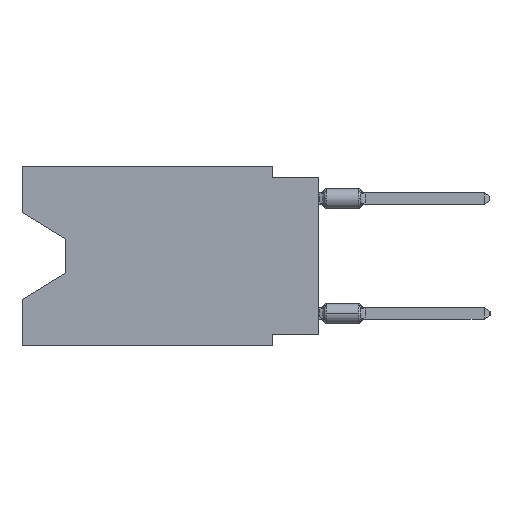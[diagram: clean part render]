
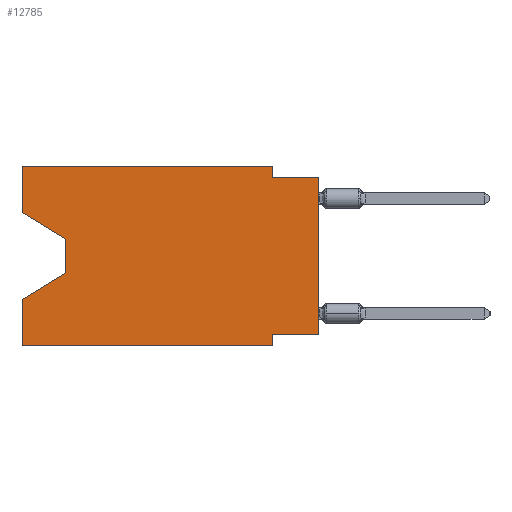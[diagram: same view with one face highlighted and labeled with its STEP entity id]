
A CAD part, left-side view. The second image highlights one B-rep face of the part: STEP entity #12785.
In plain terms, the highlighted planar face has unit normal (-1, 0, 0).
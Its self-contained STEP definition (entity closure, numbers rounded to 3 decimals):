
#31 = LINE ( 'NONE', #40084, #26179 ) ;
#1587 = VECTOR ( 'NONE', #42313, 1000. ) ;
#1826 = ORIENTED_EDGE ( 'NONE', *, *, #6703, .F. ) ;
#2196 = VERTEX_POINT ( 'NONE', #48618 ) ;
#2496 = VERTEX_POINT ( 'NONE', #7044 ) ;
#2549 = VERTEX_POINT ( 'NONE', #28681 ) ;
#4661 = DIRECTION ( 'NONE',  ( 0., -1., 0. ) ) ;
#5457 = ORIENTED_EDGE ( 'NONE', *, *, #55264, .T. ) ;
#5834 = DIRECTION ( 'NONE',  ( 0., 0., 1. ) ) ;
#6442 = VECTOR ( 'NONE', #52381, 1000. ) ;
#6459 = LINE ( 'NONE', #33902, #17753 ) ;
#6703 = EDGE_CURVE ( 'NONE', #23717, #7166, #6459, .T. ) ;
#6745 = DIRECTION ( 'NONE',  ( 0., -1., 0. ) ) ;
#7044 = CARTESIAN_POINT ( 'NONE',  ( 0., 0., -9.271 ) ) ;
#7166 = VERTEX_POINT ( 'NONE', #23918 ) ;
#8483 = LINE ( 'NONE', #8770, #37005 ) ;
#8770 = CARTESIAN_POINT ( 'NONE',  ( 0., 16.383, -9.906 ) ) ;
#9251 = DIRECTION ( 'NONE',  ( 0., -1., 0. ) ) ;
#9949 = VECTOR ( 'NONE', #29455, 1000. ) ;
#10084 = CARTESIAN_POINT ( 'NONE',  ( 0., 2.54, -9.271 ) ) ;
#10086 = ORIENTED_EDGE ( 'NONE', *, *, #16750, .F. ) ;
#10589 = ORIENTED_EDGE ( 'NONE', *, *, #33788, .F. ) ;
#11065 = ORIENTED_EDGE ( 'NONE', *, *, #12169, .T. ) ;
#11850 = VERTEX_POINT ( 'NONE', #42985 ) ;
#12040 = EDGE_CURVE ( 'NONE', #2496, #49996, #18697, .T. ) ;
#12117 = EDGE_CURVE ( 'NONE', #20123, #30701, #14608, .T. ) ;
#12169 = EDGE_CURVE ( 'NONE', #35617, #2549, #37944, .T. ) ;
#12319 = DIRECTION ( 'NONE',  ( 0., -0.855, -0.519 ) ) ;
#12782 = EDGE_CURVE ( 'NONE', #2496, #46927, #25050, .T. ) ;
#12785 = ADVANCED_FACE ( 'NONE', ( #55509 ), #16296, .F. ) ;
#14608 = LINE ( 'NONE', #41763, #45422 ) ;
#15513 = CARTESIAN_POINT ( 'NONE',  ( 0., 16.383, 0. ) ) ;
#16296 = PLANE ( 'NONE',  #34241 ) ;
#16750 = EDGE_CURVE ( 'NONE', #46927, #11850, #44417, .T. ) ;
#17237 = CARTESIAN_POINT ( 'NONE',  ( 0., 2.54, -0.635 ) ) ;
#17753 = VECTOR ( 'NONE', #6745, 1000. ) ;
#18697 = LINE ( 'NONE', #54401, #20220 ) ;
#19519 = DIRECTION ( 'NONE',  ( 1., 0., 0. ) ) ;
#20123 = VERTEX_POINT ( 'NONE', #31411 ) ;
#20220 = VECTOR ( 'NONE', #5834, 1000. ) ;
#20280 = EDGE_CURVE ( 'NONE', #7166, #43004, #31, .T. ) ;
#20502 = LINE ( 'NONE', #48001, #32930 ) ;
#22540 = EDGE_CURVE ( 'NONE', #2196, #23717, #42379, .T. ) ;
#23717 = VERTEX_POINT ( 'NONE', #15513 ) ;
#23875 = ORIENTED_EDGE ( 'NONE', *, *, #20280, .F. ) ;
#23899 = CARTESIAN_POINT ( 'NONE',  ( 0., 16.383, 0. ) ) ;
#23918 = CARTESIAN_POINT ( 'NONE',  ( 0., 2.54, 0. ) ) ;
#24478 = DIRECTION ( 'NONE',  ( 0., 0., -1. ) ) ;
#24579 = EDGE_CURVE ( 'NONE', #2196, #35617, #20502, .T. ) ;
#25050 = LINE ( 'NONE', #42595, #1587 ) ;
#25180 = CARTESIAN_POINT ( 'NONE',  ( 0., 16.383, -7.36 ) ) ;
#26179 = VECTOR ( 'NONE', #44776, 1000. ) ;
#28681 = CARTESIAN_POINT ( 'NONE',  ( 0., 13.97, -5.893 ) ) ;
#29258 = VECTOR ( 'NONE', #9251, 1000. ) ;
#29455 = DIRECTION ( 'NONE',  ( 0., 0., -1. ) ) ;
#30701 = VERTEX_POINT ( 'NONE', #25180 ) ;
#30786 = ORIENTED_EDGE ( 'NONE', *, *, #12117, .F. ) ;
#31411 = CARTESIAN_POINT ( 'NONE',  ( 0., 16.383, -9.906 ) ) ;
#32930 = VECTOR ( 'NONE', #12319, 1000. ) ;
#33788 = EDGE_CURVE ( 'NONE', #43004, #49996, #49308, .T. ) ;
#33902 = CARTESIAN_POINT ( 'NONE',  ( 0., 16.383, 0. ) ) ;
#34241 = AXIS2_PLACEMENT_3D ( 'NONE', #23899, #19519, #24478 ) ;
#34462 = DIRECTION ( 'NONE',  ( 0., 0., 1. ) ) ;
#35617 = VERTEX_POINT ( 'NONE', #55090 ) ;
#37005 = VECTOR ( 'NONE', #4661, 1000. ) ;
#37944 = LINE ( 'NONE', #43214, #9949 ) ;
#38611 = LINE ( 'NONE', #38900, #6442 ) ;
#38900 = CARTESIAN_POINT ( 'NONE',  ( 0., 13.97, -5.893 ) ) ;
#39990 = ORIENTED_EDGE ( 'NONE', *, *, #12782, .F. ) ;
#40084 = CARTESIAN_POINT ( 'NONE',  ( 0., 2.54, 0. ) ) ;
#40630 = DIRECTION ( 'NONE',  ( 0., 0., 1. ) ) ;
#41763 = CARTESIAN_POINT ( 'NONE',  ( 0., 16.383, 0. ) ) ;
#42313 = DIRECTION ( 'NONE',  ( 0., 1., 0. ) ) ;
#42379 = LINE ( 'NONE', #43250, #44149 ) ;
#42595 = CARTESIAN_POINT ( 'NONE',  ( 0., 0., -9.271 ) ) ;
#42985 = CARTESIAN_POINT ( 'NONE',  ( 0., 2.54, -9.906 ) ) ;
#43004 = VERTEX_POINT ( 'NONE', #17237 ) ;
#43214 = CARTESIAN_POINT ( 'NONE',  ( 0., 13.97, -4.013 ) ) ;
#43250 = CARTESIAN_POINT ( 'NONE',  ( 0., 16.383, 0. ) ) ;
#44149 = VECTOR ( 'NONE', #34462, 1000. ) ;
#44417 = LINE ( 'NONE', #48528, #51289 ) ;
#44776 = DIRECTION ( 'NONE',  ( 0., 0., -1. ) ) ;
#45422 = VECTOR ( 'NONE', #40630, 1000. ) ;
#46927 = VERTEX_POINT ( 'NONE', #10084 ) ;
#47626 = EDGE_CURVE ( 'NONE', #2549, #30701, #38611, .T. ) ;
#48001 = CARTESIAN_POINT ( 'NONE',  ( 0., 16.383, -2.546 ) ) ;
#48528 = CARTESIAN_POINT ( 'NONE',  ( 0., 2.54, -9.906 ) ) ;
#48618 = CARTESIAN_POINT ( 'NONE',  ( 0., 16.383, -2.546 ) ) ;
#49308 = LINE ( 'NONE', #57515, #29258 ) ;
#49441 = ORIENTED_EDGE ( 'NONE', *, *, #24579, .T. ) ;
#49641 = ORIENTED_EDGE ( 'NONE', *, *, #12040, .T. ) ;
#49996 = VERTEX_POINT ( 'NONE', #51877 ) ;
#51289 = VECTOR ( 'NONE', #53798, 1000. ) ;
#51636 = ORIENTED_EDGE ( 'NONE', *, *, #47626, .T. ) ;
#51877 = CARTESIAN_POINT ( 'NONE',  ( 0., 0., -0.635 ) ) ;
#52381 = DIRECTION ( 'NONE',  ( 0., 0.855, -0.519 ) ) ;
#53798 = DIRECTION ( 'NONE',  ( 0., 0., -1. ) ) ;
#54401 = CARTESIAN_POINT ( 'NONE',  ( 0., 0., 0. ) ) ;
#55090 = CARTESIAN_POINT ( 'NONE',  ( 0., 13.97, -4.013 ) ) ;
#55264 = EDGE_CURVE ( 'NONE', #20123, #11850, #8483, .T. ) ;
#55509 = FACE_OUTER_BOUND ( 'NONE', #57440, .T. ) ;
#57440 = EDGE_LOOP ( 'NONE', ( #49441, #11065, #51636, #30786, #5457, #10086, #39990, #49641, #10589, #23875, #1826, #57619 ) ) ;
#57515 = CARTESIAN_POINT ( 'NONE',  ( 0., 0., -0.635 ) ) ;
#57619 = ORIENTED_EDGE ( 'NONE', *, *, #22540, .F. ) ;
